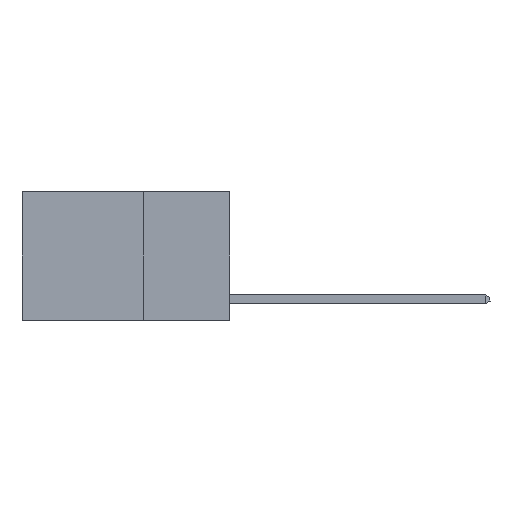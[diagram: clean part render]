
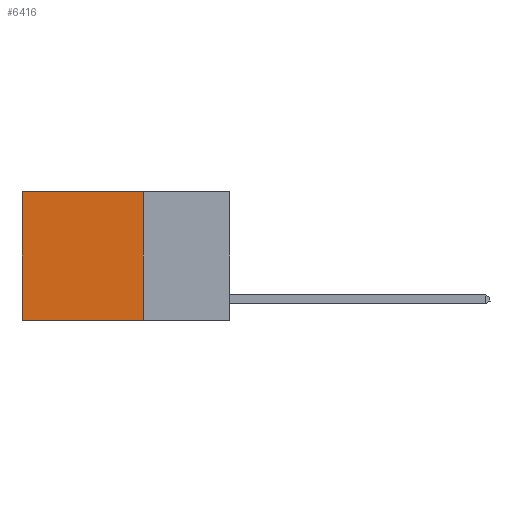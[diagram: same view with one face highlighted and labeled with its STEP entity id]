
A CAD part, left-side view. The second image highlights one B-rep face of the part: STEP entity #6416.
In plain terms, the highlighted planar face has unit normal (-1, 0, 0).
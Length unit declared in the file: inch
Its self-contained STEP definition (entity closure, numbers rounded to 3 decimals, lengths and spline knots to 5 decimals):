
#86 = EDGE_LOOP ( 'NONE', ( #1844, #1989, #2030, #2062 ) ) ;
#628 = DIRECTION ( 'NONE',  ( 0., 0., -1. ) ) ;
#744 = VERTEX_POINT ( 'NONE', #3846 ) ;
#903 = CARTESIAN_POINT ( 'NONE',  ( 0.2625, 0.6, 0. ) ) ;
#951 = LINE ( 'NONE', #903, #2908 ) ;
#1160 = FACE_OUTER_BOUND ( 'NONE', #86, .T. ) ;
#1506 = CARTESIAN_POINT ( 'NONE',  ( 0.2625, 0.25, 0. ) ) ;
#1620 = CARTESIAN_POINT ( 'NONE',  ( 0.2625, 0.25, 0. ) ) ;
#1644 = EDGE_CURVE ( 'NONE', #5427, #3361, #951, .T. ) ;
#1844 = ORIENTED_EDGE ( 'NONE', *, *, #1644, .T. ) ;
#1989 = ORIENTED_EDGE ( 'NONE', *, *, #4842, .F. ) ;
#2030 = ORIENTED_EDGE ( 'NONE', *, *, #8851, .F. ) ;
#2062 = ORIENTED_EDGE ( 'NONE', *, *, #3499, .T. ) ;
#2729 = CARTESIAN_POINT ( 'NONE',  ( 0.2625, 0.6, 0. ) ) ;
#2908 = VECTOR ( 'NONE', #628, 39.37008 ) ;
#3215 = VERTEX_POINT ( 'NONE', #9639 ) ;
#3265 = CARTESIAN_POINT ( 'NONE',  ( 0.2625, 0.25, 0. ) ) ;
#3361 = VERTEX_POINT ( 'NONE', #8967 ) ;
#3445 = DIRECTION ( 'NONE',  ( 0., 0., -1. ) ) ;
#3499 = EDGE_CURVE ( 'NONE', #3215, #5427, #9687, .T. ) ;
#3846 = CARTESIAN_POINT ( 'NONE',  ( 0.2625, 0.25, -0.37 ) ) ;
#4346 = LINE ( 'NONE', #8826, #8997 ) ;
#4842 = EDGE_CURVE ( 'NONE', #744, #3361, #4346, .T. ) ;
#5269 = VECTOR ( 'NONE', #11479, 39.37008 ) ;
#5427 = VERTEX_POINT ( 'NONE', #2729 ) ;
#5562 = LINE ( 'NONE', #3265, #5269 ) ;
#6416 = ADVANCED_FACE ( 'NONE', ( #1160 ), #11596, .F. ) ;
#7343 = VECTOR ( 'NONE', #10867, 39.37008 ) ;
#8826 = CARTESIAN_POINT ( 'NONE',  ( 0.2625, 0.25, -0.37 ) ) ;
#8851 = EDGE_CURVE ( 'NONE', #3215, #744, #5562, .T. ) ;
#8853 = AXIS2_PLACEMENT_3D ( 'NONE', #1506, #9027, #3445 ) ;
#8967 = CARTESIAN_POINT ( 'NONE',  ( 0.2625, 0.6, -0.37 ) ) ;
#8997 = VECTOR ( 'NONE', #9676, 39.37008 ) ;
#9027 = DIRECTION ( 'NONE',  ( 1., 0., 0. ) ) ;
#9639 = CARTESIAN_POINT ( 'NONE',  ( 0.2625, 0.25, 0. ) ) ;
#9676 = DIRECTION ( 'NONE',  ( 0., 1., 0. ) ) ;
#9687 = LINE ( 'NONE', #1620, #7343 ) ;
#10867 = DIRECTION ( 'NONE',  ( 0., 1., 0. ) ) ;
#11479 = DIRECTION ( 'NONE',  ( 0., 0., -1. ) ) ;
#11596 = PLANE ( 'NONE',  #8853 ) ;
